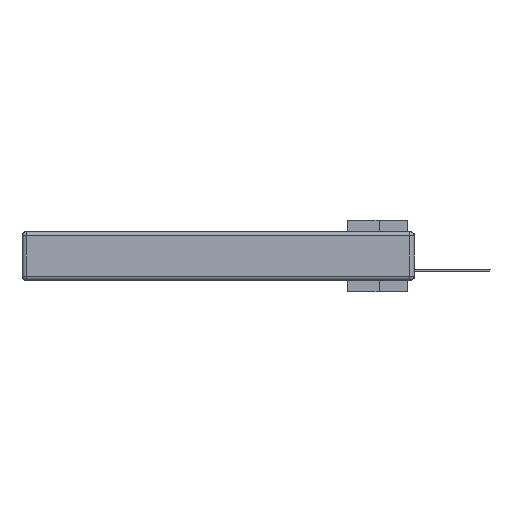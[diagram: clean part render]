
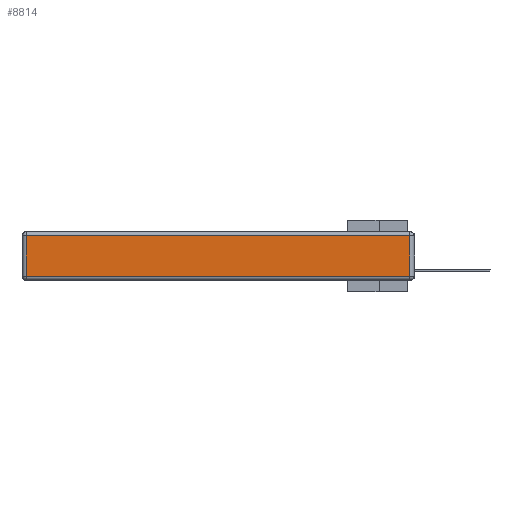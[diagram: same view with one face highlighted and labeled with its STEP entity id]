
A CAD part, left-side view. The second image highlights one B-rep face of the part: STEP entity #8814.
In plain terms, the highlighted planar face has unit normal (-1, 0, 0).
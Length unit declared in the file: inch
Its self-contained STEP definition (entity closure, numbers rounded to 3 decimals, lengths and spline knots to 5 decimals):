
#1346 = DIRECTION ( 'NONE',  ( 0., -1., 0. ) ) ;
#2878 = LINE ( 'NONE', #11633, #26628 ) ;
#3876 = EDGE_LOOP ( 'NONE', ( #18047, #6143, #24459, #26863 ) ) ;
#4830 = VERTEX_POINT ( 'NONE', #13233 ) ;
#5373 = DIRECTION ( 'NONE',  ( 0., 1., 0. ) ) ;
#5671 = CARTESIAN_POINT ( 'NONE',  ( 0., 0., -0.313 ) ) ;
#5851 = DIRECTION ( 'NONE',  ( 0., 0., -1. ) ) ;
#5881 = LINE ( 'NONE', #27894, #9092 ) ;
#6143 = ORIENTED_EDGE ( 'NONE', *, *, #9836, .T. ) ;
#6206 = VECTOR ( 'NONE', #5373, 39.37008 ) ;
#7253 = CARTESIAN_POINT ( 'NONE',  ( 0., 2.75, -0.03 ) ) ;
#8558 = VERTEX_POINT ( 'NONE', #19968 ) ;
#8814 = ADVANCED_FACE ( 'NONE', ( #14342 ), #12177, .T. ) ;
#9092 = VECTOR ( 'NONE', #18956, 39.37008 ) ;
#9836 = EDGE_CURVE ( 'NONE', #13078, #8558, #5881, .T. ) ;
#11314 = AXIS2_PLACEMENT_3D ( 'NONE', #19076, #23259, #17060 ) ;
#11627 = VECTOR ( 'NONE', #1346, 39.37008 ) ;
#11633 = CARTESIAN_POINT ( 'NONE',  ( 0., 2.72, -0.343 ) ) ;
#12177 = PLANE ( 'NONE',  #11314 ) ;
#12995 = VERTEX_POINT ( 'NONE', #19119 ) ;
#13078 = VERTEX_POINT ( 'NONE', #15658 ) ;
#13233 = CARTESIAN_POINT ( 'NONE',  ( 0., 2.72, -0.313 ) ) ;
#14342 = FACE_OUTER_BOUND ( 'NONE', #3876, .T. ) ;
#14898 = EDGE_CURVE ( 'NONE', #4830, #13078, #25524, .T. ) ;
#15658 = CARTESIAN_POINT ( 'NONE',  ( 0., 0.03, -0.313 ) ) ;
#16022 = LINE ( 'NONE', #7253, #6206 ) ;
#17060 = DIRECTION ( 'NONE',  ( 0., 0., 1. ) ) ;
#18047 = ORIENTED_EDGE ( 'NONE', *, *, #14898, .T. ) ;
#18956 = DIRECTION ( 'NONE',  ( 0., 0., 1. ) ) ;
#19076 = CARTESIAN_POINT ( 'NONE',  ( 0., 0., -0.343 ) ) ;
#19119 = CARTESIAN_POINT ( 'NONE',  ( 0., 2.72, -0.03 ) ) ;
#19836 = EDGE_CURVE ( 'NONE', #8558, #12995, #16022, .T. ) ;
#19968 = CARTESIAN_POINT ( 'NONE',  ( 0., 0.03, -0.03 ) ) ;
#23259 = DIRECTION ( 'NONE',  ( -1., 0., 0. ) ) ;
#24459 = ORIENTED_EDGE ( 'NONE', *, *, #19836, .T. ) ;
#25524 = LINE ( 'NONE', #5671, #11627 ) ;
#26157 = EDGE_CURVE ( 'NONE', #12995, #4830, #2878, .T. ) ;
#26628 = VECTOR ( 'NONE', #5851, 39.37008 ) ;
#26863 = ORIENTED_EDGE ( 'NONE', *, *, #26157, .T. ) ;
#27894 = CARTESIAN_POINT ( 'NONE',  ( 0., 0.03, -0.343 ) ) ;
